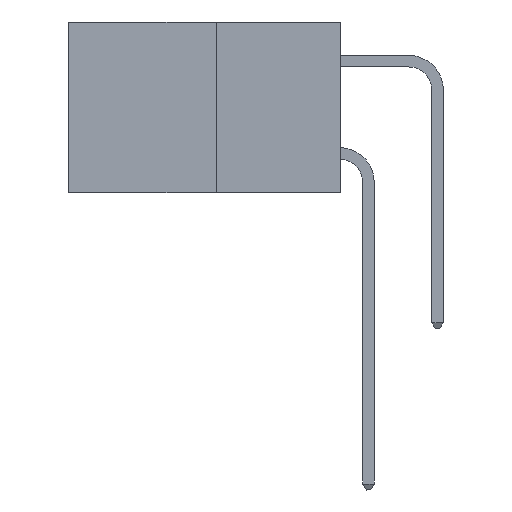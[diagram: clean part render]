
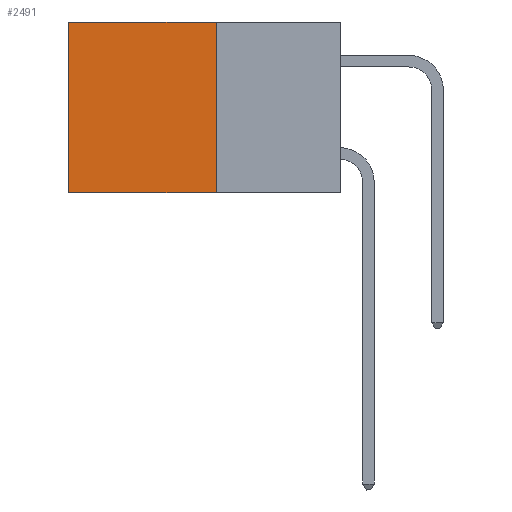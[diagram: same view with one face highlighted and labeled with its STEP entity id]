
A CAD part, left-side view. The second image highlights one B-rep face of the part: STEP entity #2491.
In plain terms, the highlighted planar face has unit normal (-1, 0, 0).
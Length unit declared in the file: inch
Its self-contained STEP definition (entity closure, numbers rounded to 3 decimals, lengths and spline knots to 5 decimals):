
#411 = CARTESIAN_POINT ( 'NONE',  ( 0.277, 0.59, -0.37 ) ) ;
#771 = EDGE_CURVE ( 'NONE', #3563, #16166, #9637, .T. ) ;
#1978 = VECTOR ( 'NONE', #21307, 39.37008 ) ;
#2363 = ORIENTED_EDGE ( 'NONE', *, *, #6953, .F. ) ;
#2491 = ADVANCED_FACE ( 'NONE', ( #4372 ), #2934, .F. ) ;
#2934 = PLANE ( 'NONE',  #8555 ) ;
#3563 = VERTEX_POINT ( 'NONE', #22318 ) ;
#4366 = CARTESIAN_POINT ( 'NONE',  ( 0.277, 0.59, 0. ) ) ;
#4372 = FACE_OUTER_BOUND ( 'NONE', #15296, .T. ) ;
#5856 = VERTEX_POINT ( 'NONE', #411 ) ;
#6067 = ORIENTED_EDGE ( 'NONE', *, *, #771, .T. ) ;
#6680 = VECTOR ( 'NONE', #11096, 39.37008 ) ;
#6953 = EDGE_CURVE ( 'NONE', #13692, #5856, #15947, .T. ) ;
#7418 = CARTESIAN_POINT ( 'NONE',  ( 0.277, 0.27, -0.37 ) ) ;
#7669 = CARTESIAN_POINT ( 'NONE',  ( 0.277, 0.59, -0.37 ) ) ;
#7946 = VECTOR ( 'NONE', #19092, 39.37008 ) ;
#8555 = AXIS2_PLACEMENT_3D ( 'NONE', #19090, #12076, #17933 ) ;
#8975 = ORIENTED_EDGE ( 'NONE', *, *, #10751, .T. ) ;
#9637 = LINE ( 'NONE', #20800, #18299 ) ;
#10104 = CARTESIAN_POINT ( 'NONE',  ( 0.277, 0.27, -0.37 ) ) ;
#10751 = EDGE_CURVE ( 'NONE', #16166, #5856, #16489, .T. ) ;
#11096 = DIRECTION ( 'NONE',  ( 0., 0., -1. ) ) ;
#11978 = DIRECTION ( 'NONE',  ( 0., 1., 0. ) ) ;
#12076 = DIRECTION ( 'NONE',  ( 1., 0., 0. ) ) ;
#12581 = LINE ( 'NONE', #17376, #7946 ) ;
#13692 = VERTEX_POINT ( 'NONE', #10104 ) ;
#13845 = EDGE_CURVE ( 'NONE', #3563, #13692, #12581, .T. ) ;
#15296 = EDGE_LOOP ( 'NONE', ( #8975, #2363, #18039, #6067 ) ) ;
#15947 = LINE ( 'NONE', #7418, #1978 ) ;
#16166 = VERTEX_POINT ( 'NONE', #4366 ) ;
#16489 = LINE ( 'NONE', #7669, #6680 ) ;
#17376 = CARTESIAN_POINT ( 'NONE',  ( 0.277, 0.27, -0.37 ) ) ;
#17933 = DIRECTION ( 'NONE',  ( 0., 0., -1. ) ) ;
#18039 = ORIENTED_EDGE ( 'NONE', *, *, #13845, .F. ) ;
#18299 = VECTOR ( 'NONE', #11978, 39.37008 ) ;
#19090 = CARTESIAN_POINT ( 'NONE',  ( 0.277, 0.27, -0.37 ) ) ;
#19092 = DIRECTION ( 'NONE',  ( 0., 0., -1. ) ) ;
#20800 = CARTESIAN_POINT ( 'NONE',  ( 0.277, 0.27, 0. ) ) ;
#21307 = DIRECTION ( 'NONE',  ( 0., 1., 0. ) ) ;
#22318 = CARTESIAN_POINT ( 'NONE',  ( 0.277, 0.27, 0. ) ) ;
